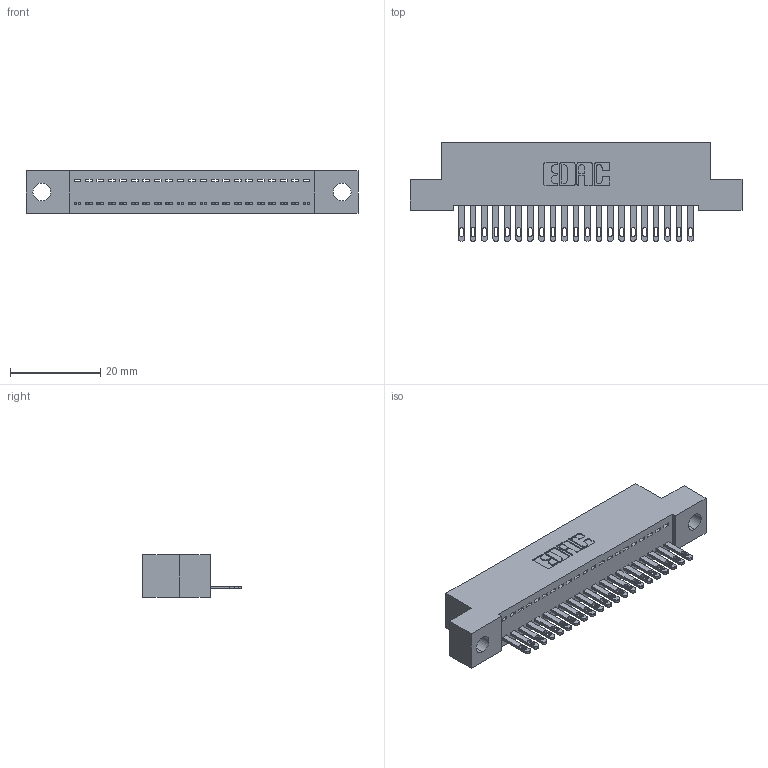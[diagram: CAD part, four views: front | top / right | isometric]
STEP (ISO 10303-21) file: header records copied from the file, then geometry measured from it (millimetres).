
FILE_DESCRIPTION (( 'STEP AP203' ), '1' );
FILE_NAME ('342-021-500-104.STEP', '2018-08-10T23:34:17', ( '' ), ( '' ), 'SwSTEP 2.0', 'SolidWorks 2016', '' );
FILE_SCHEMA (( 'CONFIG_CONTROL_DESIGN' ));
Length unit declared in the file: inch
Products named in the file (3): 345-292-001_345-293-100; 342-021-500-104; 342 Part_.156 TH
Assembly tree (22 placements, depth 2):
  342-021-500-104
    342 Part_.156 TH
    345-292-001_345-293-100  x21
Bounding box: 73.66 x 21.85 x 9.4 mm (x, y, z)
Volume: 6307.1 mm3; surface area: 8729.8 mm2
Topology: 22 solids, 22 shells, 1244 faces, 3827 edges, 2550 vertices
Faces by surface type: plane 822, cylinder 422
Entity records: 15355 total; most frequent: CARTESIAN_POINT 2657, ORIENTED_EDGE 2614, DIRECTION 2285, EDGE_CURVE 1307, LINE 1175, VECTOR 1175, VERTEX_POINT 870, AXIS2_PLACEMENT_3D 555
